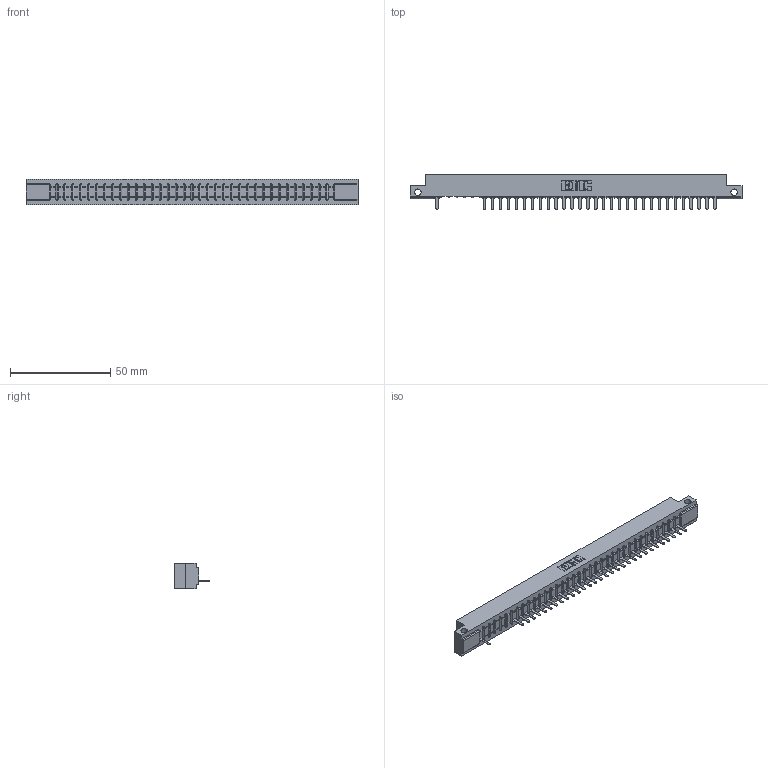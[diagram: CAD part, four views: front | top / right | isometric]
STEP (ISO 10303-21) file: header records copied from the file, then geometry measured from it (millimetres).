
FILE_DESCRIPTION (( 'STEP AP203' ), '1' );
FILE_NAME ('357-036-521-112.STEP', '2018-08-10T05:42:04', ( '' ), ( '' ), 'SwSTEP 2.0', 'SolidWorks 2016', '' );
FILE_SCHEMA (( 'CONFIG_CONTROL_DESIGN' ));
Length unit declared in the file: inch
Products named in the file (3): 307 Part_.128 Dia Side Mounting Holes; 307-290-002_521; 357-036-521-112
Assembly tree (32 placements, depth 2):
  357-036-521-112
    307 Part_.128 Dia Side Mounting Holes
    307-290-002_521  x31
Bounding box: 165.66 x 17.42 x 12.7 mm (x, y, z)
Volume: 17397.9 mm3; surface area: 20811.5 mm2
Topology: 32 solids, 32 shells, 2549 faces, 7835 edges, 5122 vertices
Faces by surface type: plane 1525, cylinder 950, sphere 74
Entity records: 32162 total; most frequent: CARTESIAN_POINT 5447, ORIENTED_EDGE 5442, DIRECTION 5289, EDGE_CURVE 2721, LINE 2081, VECTOR 2081, VERTEX_POINT 1762, AXIS2_PLACEMENT_3D 1604
